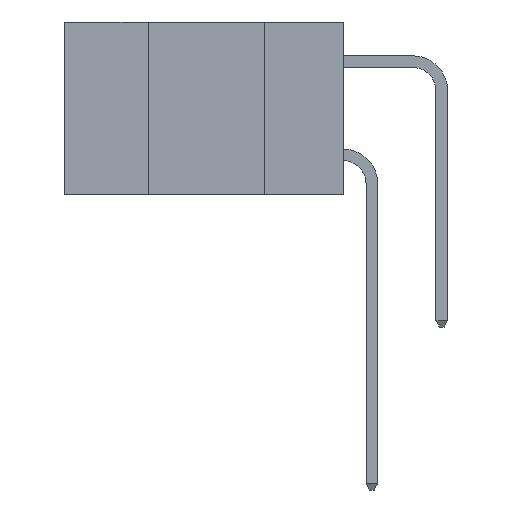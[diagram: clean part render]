
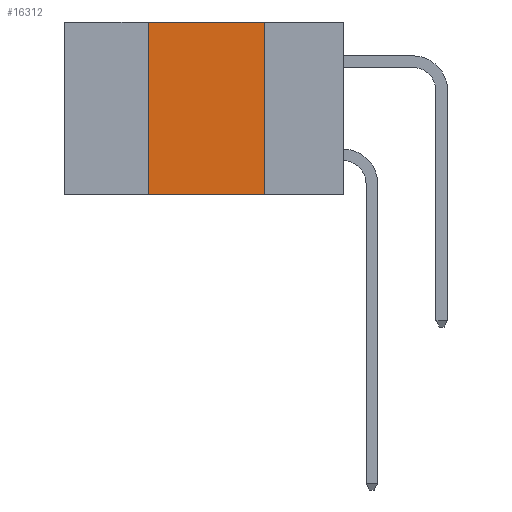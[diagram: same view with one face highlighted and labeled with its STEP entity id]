
A CAD part, left-side view. The second image highlights one B-rep face of the part: STEP entity #16312.
In plain terms, the highlighted planar face has unit normal (-1, 0, 0).
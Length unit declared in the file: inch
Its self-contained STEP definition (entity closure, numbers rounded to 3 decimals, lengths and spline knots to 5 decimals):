
#1728 = VERTEX_POINT ( 'NONE', #12510 ) ;
#2073 = CARTESIAN_POINT ( 'NONE',  ( 0., 0.42, -0.37 ) ) ;
#2077 = VERTEX_POINT ( 'NONE', #6990 ) ;
#2943 = VECTOR ( 'NONE', #9604, 39.37008 ) ;
#3436 = LINE ( 'NONE', #9896, #2943 ) ;
#3645 = PLANE ( 'NONE',  #19018 ) ;
#4249 = VECTOR ( 'NONE', #6069, 39.37008 ) ;
#4400 = CARTESIAN_POINT ( 'NONE',  ( 0., 0.17, -0.37 ) ) ;
#4479 = CARTESIAN_POINT ( 'NONE',  ( 0., 0.6, 0. ) ) ;
#5281 = ORIENTED_EDGE ( 'NONE', *, *, #15282, .F. ) ;
#5994 = ORIENTED_EDGE ( 'NONE', *, *, #14900, .F. ) ;
#6069 = DIRECTION ( 'NONE',  ( 0., -1., 0. ) ) ;
#6806 = DIRECTION ( 'NONE',  ( 1., 0., 0. ) ) ;
#6883 = ORIENTED_EDGE ( 'NONE', *, *, #7642, .T. ) ;
#6952 = VECTOR ( 'NONE', #19956, 39.37008 ) ;
#6990 = CARTESIAN_POINT ( 'NONE',  ( 0., 0.17, -0.37 ) ) ;
#7642 = EDGE_CURVE ( 'NONE', #16306, #2077, #3436, .T. ) ;
#7933 = VECTOR ( 'NONE', #14642, 39.37008 ) ;
#8417 = LINE ( 'NONE', #11504, #7933 ) ;
#8421 = LINE ( 'NONE', #4479, #4249 ) ;
#9604 = DIRECTION ( 'NONE',  ( 0., -1., 0. ) ) ;
#9883 = ORIENTED_EDGE ( 'NONE', *, *, #15943, .F. ) ;
#9896 = CARTESIAN_POINT ( 'NONE',  ( 0., 0.6, -0.37 ) ) ;
#11068 = LINE ( 'NONE', #4400, #6952 ) ;
#11504 = CARTESIAN_POINT ( 'NONE',  ( 0., 0.42, -0.37 ) ) ;
#12510 = CARTESIAN_POINT ( 'NONE',  ( 0., 0.42, 0. ) ) ;
#13107 = CARTESIAN_POINT ( 'NONE',  ( 0., 0.17, 0. ) ) ;
#14120 = EDGE_LOOP ( 'NONE', ( #5994, #9883, #5281, #6883 ) ) ;
#14642 = DIRECTION ( 'NONE',  ( 0., 0., 1. ) ) ;
#14900 = EDGE_CURVE ( 'NONE', #16992, #2077, #11068, .T. ) ;
#15282 = EDGE_CURVE ( 'NONE', #16306, #1728, #8417, .T. ) ;
#15943 = EDGE_CURVE ( 'NONE', #1728, #16992, #8421, .T. ) ;
#16079 = CARTESIAN_POINT ( 'NONE',  ( 0., 0.6, 0. ) ) ;
#16306 = VERTEX_POINT ( 'NONE', #2073 ) ;
#16312 = ADVANCED_FACE ( 'NONE', ( #18103 ), #3645, .F. ) ;
#16992 = VERTEX_POINT ( 'NONE', #13107 ) ;
#17646 = DIRECTION ( 'NONE',  ( 0., 0., -1. ) ) ;
#18103 = FACE_OUTER_BOUND ( 'NONE', #14120, .T. ) ;
#19018 = AXIS2_PLACEMENT_3D ( 'NONE', #16079, #6806, #17646 ) ;
#19956 = DIRECTION ( 'NONE',  ( 0., 0., -1. ) ) ;
